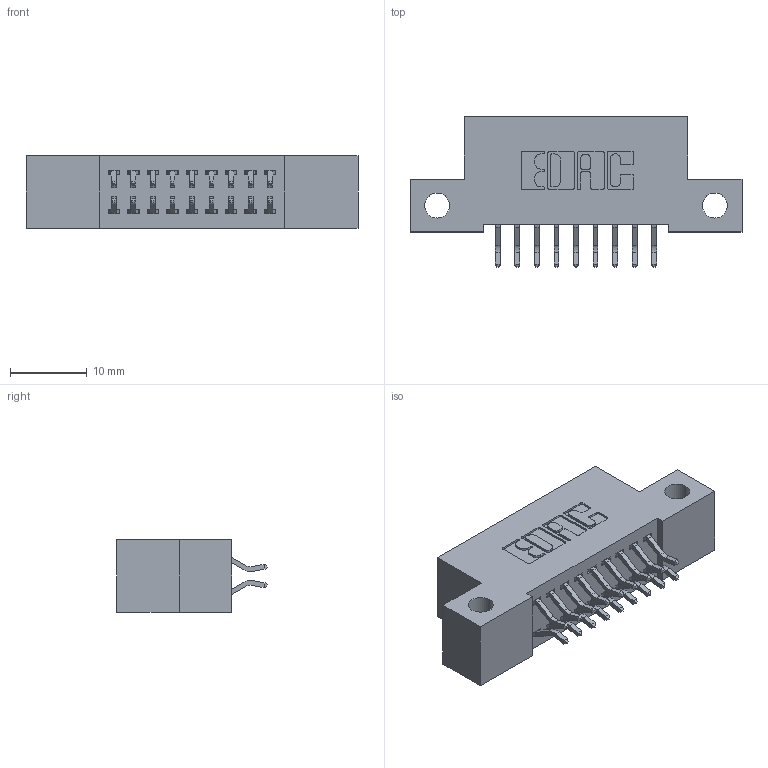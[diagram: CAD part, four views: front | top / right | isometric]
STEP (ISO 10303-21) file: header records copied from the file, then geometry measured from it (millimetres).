
FILE_DESCRIPTION (( 'STEP AP203' ), '1' );
FILE_NAME ('342-018-556-212.STEP', '2018-08-10T21:46:49', ( '' ), ( '' ), 'SwSTEP 2.0', 'SolidWorks 2016', '' );
FILE_SCHEMA (( 'CONFIG_CONTROL_DESIGN' ));
Length unit declared in the file: inch
Products named in the file (3): 342 Part_Side Mount; 345-292-001_556 Tail; 342-018-556-212
Assembly tree (19 placements, depth 2):
  342-018-556-212
    342 Part_Side Mount
    345-292-001_556 Tail  x18
Bounding box: 43.18 x 19.58 x 9.4 mm (x, y, z)
Volume: 3649.1 mm3; surface area: 4949.5 mm2
Topology: 19 solids, 19 shells, 1154 faces, 3413 edges, 2250 vertices
Faces by surface type: plane 786, cylinder 368
Entity records: 10149 total; most frequent: CARTESIAN_POINT 1734, ORIENTED_EDGE 1658, DIRECTION 1529, EDGE_CURVE 829, LINE 693, VECTOR 693, VERTEX_POINT 550, AXIS2_PLACEMENT_3D 418
